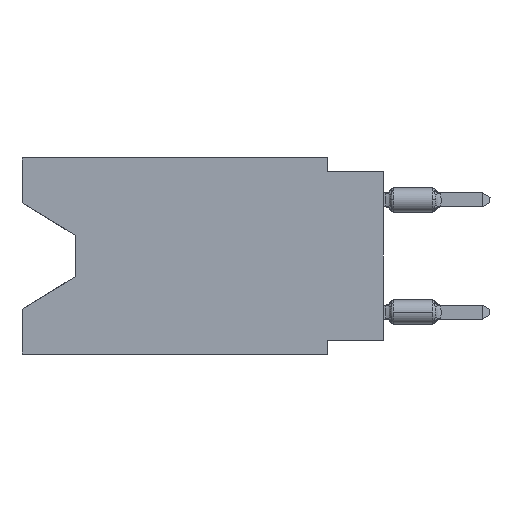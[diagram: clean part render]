
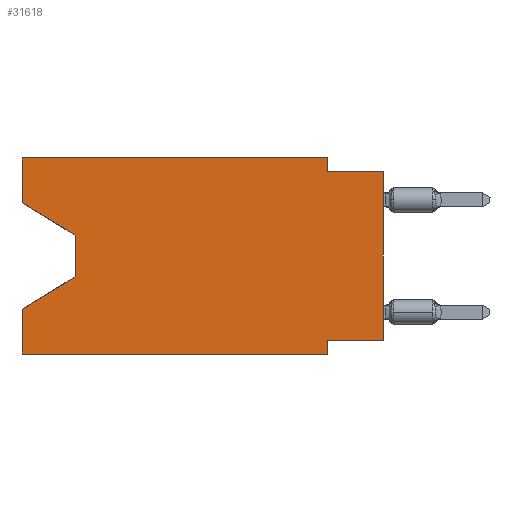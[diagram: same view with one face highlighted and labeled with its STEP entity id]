
A CAD part, left-side view. The second image highlights one B-rep face of the part: STEP entity #31618.
In plain terms, the highlighted planar face has unit normal (-1, 0, 0).
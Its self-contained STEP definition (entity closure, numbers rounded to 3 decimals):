
#182 = CARTESIAN_POINT ( 'NONE',  ( 0., 13.97, -5.385 ) ) ;
#636 = CARTESIAN_POINT ( 'NONE',  ( 0., 2.54, -8.89 ) ) ;
#2214 = CARTESIAN_POINT ( 'NONE',  ( 0., 2.54, -8.89 ) ) ;
#2558 = CARTESIAN_POINT ( 'NONE',  ( 0., 16.383, -8.89 ) ) ;
#2613 = CARTESIAN_POINT ( 'NONE',  ( 0., 16.383, 0. ) ) ;
#2655 = EDGE_CURVE ( 'NONE', #36501, #42587, #6581, .T. ) ;
#3002 = CARTESIAN_POINT ( 'NONE',  ( 0., 2.54, 0. ) ) ;
#3069 = EDGE_CURVE ( 'NONE', #40215, #6465, #5838, .T. ) ;
#3684 = EDGE_CURVE ( 'NONE', #36262, #9154, #44763, .T. ) ;
#3905 = ORIENTED_EDGE ( 'NONE', *, *, #44243, .F. ) ;
#4703 = CARTESIAN_POINT ( 'NONE',  ( 0., 13.97, -3.505 ) ) ;
#4746 = EDGE_CURVE ( 'NONE', #43076, #9154, #20239, .T. ) ;
#5394 = VERTEX_POINT ( 'NONE', #28758 ) ;
#5598 = DIRECTION ( 'NONE',  ( 0., 0., -1. ) ) ;
#5838 = LINE ( 'NONE', #30473, #8502 ) ;
#5907 = VECTOR ( 'NONE', #41047, 1000. ) ;
#6321 = VECTOR ( 'NONE', #33825, 1000. ) ;
#6465 = VERTEX_POINT ( 'NONE', #32027 ) ;
#6581 = LINE ( 'NONE', #26665, #42606 ) ;
#7890 = CARTESIAN_POINT ( 'NONE',  ( 0., 0., -0.635 ) ) ;
#8502 = VECTOR ( 'NONE', #12595, 1000. ) ;
#9021 = VERTEX_POINT ( 'NONE', #21336 ) ;
#9154 = VERTEX_POINT ( 'NONE', #636 ) ;
#9440 = ORIENTED_EDGE ( 'NONE', *, *, #27463, .F. ) ;
#10060 = VECTOR ( 'NONE', #10470, 1000. ) ;
#10234 = CARTESIAN_POINT ( 'NONE',  ( 0., 0., 0. ) ) ;
#10470 = DIRECTION ( 'NONE',  ( 0., 0., 1. ) ) ;
#10501 = CARTESIAN_POINT ( 'NONE',  ( 0., 0., -8.255 ) ) ;
#11349 = LINE ( 'NONE', #182, #16687 ) ;
#11579 = ORIENTED_EDGE ( 'NONE', *, *, #12602, .T. ) ;
#12570 = VECTOR ( 'NONE', #21367, 1000. ) ;
#12595 = DIRECTION ( 'NONE',  ( 0., -0.855, -0.519 ) ) ;
#12602 = EDGE_CURVE ( 'NONE', #6465, #5394, #19556, .T. ) ;
#12964 = CARTESIAN_POINT ( 'NONE',  ( 0., 16.383, -6.852 ) ) ;
#13261 = DIRECTION ( 'NONE',  ( 0., -1., 0. ) ) ;
#13404 = VECTOR ( 'NONE', #5598, 1000. ) ;
#14116 = EDGE_CURVE ( 'NONE', #19143, #42587, #45822, .T. ) ;
#14960 = EDGE_CURVE ( 'NONE', #43076, #43500, #20363, .T. ) ;
#15469 = FACE_OUTER_BOUND ( 'NONE', #22712, .T. ) ;
#15767 = ORIENTED_EDGE ( 'NONE', *, *, #14960, .F. ) ;
#15924 = CARTESIAN_POINT ( 'NONE',  ( 0., 16.383, -2.038 ) ) ;
#16322 = VECTOR ( 'NONE', #25166, 1000. ) ;
#16687 = VECTOR ( 'NONE', #24629, 1000. ) ;
#17362 = CARTESIAN_POINT ( 'NONE',  ( 0., 2.54, 0. ) ) ;
#18727 = ORIENTED_EDGE ( 'NONE', *, *, #38003, .T. ) ;
#18730 = DIRECTION ( 'NONE',  ( 1., 0., 0. ) ) ;
#19143 = VERTEX_POINT ( 'NONE', #43145 ) ;
#19455 = DIRECTION ( 'NONE',  ( 0., -1., 0. ) ) ;
#19556 = LINE ( 'NONE', #4703, #13404 ) ;
#20239 = LINE ( 'NONE', #2558, #23644 ) ;
#20319 = VECTOR ( 'NONE', #27250, 1000. ) ;
#20330 = ORIENTED_EDGE ( 'NONE', *, *, #3684, .F. ) ;
#20363 = LINE ( 'NONE', #34501, #6321 ) ;
#21336 = CARTESIAN_POINT ( 'NONE',  ( 0., 16.383, 0. ) ) ;
#21367 = DIRECTION ( 'NONE',  ( 0., 0., -1. ) ) ;
#22712 = EDGE_LOOP ( 'NONE', ( #29783, #11579, #18727, #15767, #41952, #20330, #34927, #28948, #29545, #9440, #29195, #3905 ) ) ;
#23644 = VECTOR ( 'NONE', #13261, 1000. ) ;
#24629 = DIRECTION ( 'NONE',  ( 0., 0.855, -0.519 ) ) ;
#25166 = DIRECTION ( 'NONE',  ( 0., 1., 0. ) ) ;
#26165 = CARTESIAN_POINT ( 'NONE',  ( 0., 16.383, 0. ) ) ;
#26665 = CARTESIAN_POINT ( 'NONE',  ( 0., 0., -0.635 ) ) ;
#26841 = AXIS2_PLACEMENT_3D ( 'NONE', #26165, #18730, #36828 ) ;
#27250 = DIRECTION ( 'NONE',  ( 0., 0., 1. ) ) ;
#27463 = EDGE_CURVE ( 'NONE', #41618, #36501, #32040, .T. ) ;
#28758 = CARTESIAN_POINT ( 'NONE',  ( 0., 13.97, -5.385 ) ) ;
#28948 = ORIENTED_EDGE ( 'NONE', *, *, #14116, .T. ) ;
#29195 = ORIENTED_EDGE ( 'NONE', *, *, #42484, .F. ) ;
#29545 = ORIENTED_EDGE ( 'NONE', *, *, #2655, .F. ) ;
#29783 = ORIENTED_EDGE ( 'NONE', *, *, #3069, .T. ) ;
#30473 = CARTESIAN_POINT ( 'NONE',  ( 0., 16.383, -2.038 ) ) ;
#30911 = CARTESIAN_POINT ( 'NONE',  ( 0., 2.54, -8.255 ) ) ;
#31618 = ADVANCED_FACE ( 'NONE', ( #15469 ), #40563, .F. ) ;
#32027 = CARTESIAN_POINT ( 'NONE',  ( 0., 13.97, -3.505 ) ) ;
#32040 = LINE ( 'NONE', #3002, #12570 ) ;
#33825 = DIRECTION ( 'NONE',  ( 0., 0., 1. ) ) ;
#34501 = CARTESIAN_POINT ( 'NONE',  ( 0., 16.383, 0. ) ) ;
#34927 = ORIENTED_EDGE ( 'NONE', *, *, #42050, .F. ) ;
#35524 = DIRECTION ( 'NONE',  ( 0., -1., 0. ) ) ;
#36262 = VERTEX_POINT ( 'NONE', #30911 ) ;
#36501 = VERTEX_POINT ( 'NONE', #43486 ) ;
#36828 = DIRECTION ( 'NONE',  ( 0., 0., -1. ) ) ;
#38003 = EDGE_CURVE ( 'NONE', #5394, #43500, #11349, .T. ) ;
#39022 = CARTESIAN_POINT ( 'NONE',  ( 0., 16.383, 0. ) ) ;
#40215 = VERTEX_POINT ( 'NONE', #15924 ) ;
#40563 = PLANE ( 'NONE',  #26841 ) ;
#40745 = VECTOR ( 'NONE', #35524, 1000. ) ;
#40777 = LINE ( 'NONE', #2613, #20319 ) ;
#41047 = DIRECTION ( 'NONE',  ( 0., 0., -1. ) ) ;
#41618 = VERTEX_POINT ( 'NONE', #17362 ) ;
#41952 = ORIENTED_EDGE ( 'NONE', *, *, #4746, .T. ) ;
#42050 = EDGE_CURVE ( 'NONE', #19143, #36262, #42588, .T. ) ;
#42484 = EDGE_CURVE ( 'NONE', #9021, #41618, #42533, .T. ) ;
#42533 = LINE ( 'NONE', #39022, #40745 ) ;
#42587 = VERTEX_POINT ( 'NONE', #7890 ) ;
#42588 = LINE ( 'NONE', #10501, #16322 ) ;
#42606 = VECTOR ( 'NONE', #19455, 1000. ) ;
#43076 = VERTEX_POINT ( 'NONE', #44088 ) ;
#43145 = CARTESIAN_POINT ( 'NONE',  ( 0., 0., -8.255 ) ) ;
#43486 = CARTESIAN_POINT ( 'NONE',  ( 0., 2.54, -0.635 ) ) ;
#43500 = VERTEX_POINT ( 'NONE', #12964 ) ;
#44088 = CARTESIAN_POINT ( 'NONE',  ( 0., 16.383, -8.89 ) ) ;
#44243 = EDGE_CURVE ( 'NONE', #40215, #9021, #40777, .T. ) ;
#44763 = LINE ( 'NONE', #2214, #5907 ) ;
#45822 = LINE ( 'NONE', #10234, #10060 ) ;
